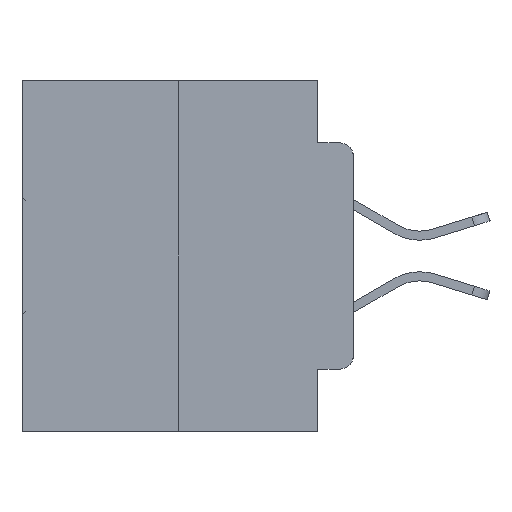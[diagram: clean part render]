
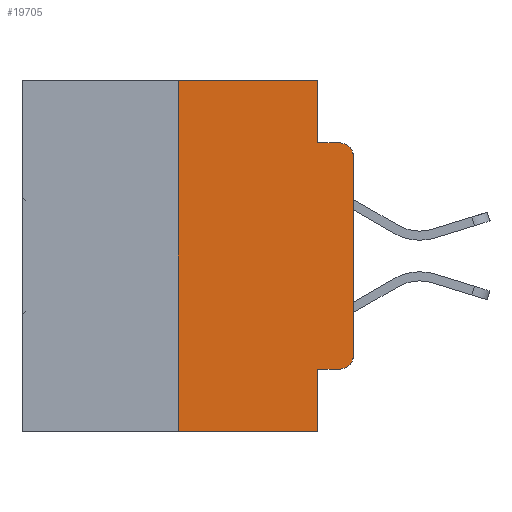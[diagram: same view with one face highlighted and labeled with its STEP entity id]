
A CAD part, left-side view. The second image highlights one B-rep face of the part: STEP entity #19705.
In plain terms, the highlighted planar face has unit normal (-1, 0, 0).
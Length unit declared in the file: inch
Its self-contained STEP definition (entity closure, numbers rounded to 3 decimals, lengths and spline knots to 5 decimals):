
#612 = VERTEX_POINT ( 'NONE', #26091 ) ;
#652 = EDGE_CURVE ( 'NONE', #20624, #612, #1993, .T. ) ;
#1341 = DIRECTION ( 'NONE',  ( 0., -1., 0. ) ) ;
#1953 = EDGE_CURVE ( 'NONE', #21382, #4278, #17547, .T. ) ;
#1993 = LINE ( 'NONE', #6471, #13071 ) ;
#2109 = CIRCLE ( 'NONE', #30244, 0.02 ) ;
#2311 = DIRECTION ( 'NONE',  ( 0., 0., -1. ) ) ;
#2316 = DIRECTION ( 'NONE',  ( 0., 0., -1. ) ) ;
#2980 = CARTESIAN_POINT ( 'NONE',  ( 0., 0.02, -0.1085 ) ) ;
#3185 = DIRECTION ( 'NONE',  ( 0., 0., 1. ) ) ;
#3675 = EDGE_CURVE ( 'NONE', #23677, #4278, #2109, .T. ) ;
#4153 = CIRCLE ( 'NONE', #27238, 0.02 ) ;
#4278 = VERTEX_POINT ( 'NONE', #30336 ) ;
#4322 = LINE ( 'NONE', #11674, #23348 ) ;
#4715 = VERTEX_POINT ( 'NONE', #14720 ) ;
#5131 = ORIENTED_EDGE ( 'NONE', *, *, #17957, .F. ) ;
#5342 = DIRECTION ( 'NONE',  ( -1., 0., 0. ) ) ;
#5421 = EDGE_CURVE ( 'NONE', #15825, #23677, #31014, .T. ) ;
#5577 = DIRECTION ( 'NONE',  ( 0., 0., -1. ) ) ;
#5592 = ORIENTED_EDGE ( 'NONE', *, *, #652, .T. ) ;
#5945 = AXIS2_PLACEMENT_3D ( 'NONE', #31873, #17349, #2316 ) ;
#6471 = CARTESIAN_POINT ( 'NONE',  ( 0., 0.473, -0.5 ) ) ;
#6844 = ORIENTED_EDGE ( 'NONE', *, *, #29112, .F. ) ;
#7915 = ORIENTED_EDGE ( 'NONE', *, *, #24277, .T. ) ;
#8422 = ORIENTED_EDGE ( 'NONE', *, *, #25894, .F. ) ;
#9498 = DIRECTION ( 'NONE',  ( 0., -1., 0. ) ) ;
#9536 = ORIENTED_EDGE ( 'NONE', *, *, #22632, .T. ) ;
#9885 = CARTESIAN_POINT ( 'NONE',  ( 0., 0.473, 0. ) ) ;
#11056 = VECTOR ( 'NONE', #2311, 39.37008 ) ;
#11674 = CARTESIAN_POINT ( 'NONE',  ( 0., 0.051, 0. ) ) ;
#12160 = VERTEX_POINT ( 'NONE', #20663 ) ;
#12467 = VERTEX_POINT ( 'NONE', #21724 ) ;
#12592 = CARTESIAN_POINT ( 'NONE',  ( 0., 0.25, -0.5 ) ) ;
#13071 = VECTOR ( 'NONE', #14023, 39.37008 ) ;
#13383 = DIRECTION ( 'NONE',  ( 0., 0., 1. ) ) ;
#13557 = ORIENTED_EDGE ( 'NONE', *, *, #3675, .T. ) ;
#14023 = DIRECTION ( 'NONE',  ( 0., -1., 0. ) ) ;
#14187 = DIRECTION ( 'NONE',  ( 0., 0., -1. ) ) ;
#14583 = ORIENTED_EDGE ( 'NONE', *, *, #1953, .F. ) ;
#14720 = CARTESIAN_POINT ( 'NONE',  ( 0., 0.051, -0.4115 ) ) ;
#14884 = CARTESIAN_POINT ( 'NONE',  ( 0., 0.051, 0. ) ) ;
#15825 = VERTEX_POINT ( 'NONE', #22467 ) ;
#15862 = VECTOR ( 'NONE', #22148, 39.37008 ) ;
#16589 = CARTESIAN_POINT ( 'NONE',  ( 0., 0., -0.1085 ) ) ;
#17349 = DIRECTION ( 'NONE',  ( 1., 0., 0. ) ) ;
#17547 = LINE ( 'NONE', #24125, #28156 ) ;
#17957 = EDGE_CURVE ( 'NONE', #12467, #12160, #22346, .T. ) ;
#18044 = CARTESIAN_POINT ( 'NONE',  ( 0., 0.051, -0.0885 ) ) ;
#19705 = ADVANCED_FACE ( 'NONE', ( #29414 ), #29444, .F. ) ;
#20195 = CARTESIAN_POINT ( 'NONE',  ( 0., 0.02, -0.3915 ) ) ;
#20419 = DIRECTION ( 'NONE',  ( -1., 0., 0. ) ) ;
#20471 = CARTESIAN_POINT ( 'NONE',  ( 0., 0.02, -0.4115 ) ) ;
#20607 = CARTESIAN_POINT ( 'NONE',  ( 0., 0.25, 0. ) ) ;
#20624 = VERTEX_POINT ( 'NONE', #12592 ) ;
#20645 = CARTESIAN_POINT ( 'NONE',  ( 0., 0., 0. ) ) ;
#20663 = CARTESIAN_POINT ( 'NONE',  ( 0., 0.051, 0. ) ) ;
#21220 = CARTESIAN_POINT ( 'NONE',  ( 0., 0.051, -0.4115 ) ) ;
#21382 = VERTEX_POINT ( 'NONE', #18044 ) ;
#21724 = CARTESIAN_POINT ( 'NONE',  ( 0., 0.25, 0. ) ) ;
#21937 = VECTOR ( 'NONE', #1341, 39.37008 ) ;
#22148 = DIRECTION ( 'NONE',  ( 0., -1., 0. ) ) ;
#22346 = LINE ( 'NONE', #9885, #15862 ) ;
#22467 = CARTESIAN_POINT ( 'NONE',  ( 0., 0., -0.3915 ) ) ;
#22632 = EDGE_CURVE ( 'NONE', #28074, #15825, #4153, .T. ) ;
#22663 = DIRECTION ( 'NONE',  ( 0., 0., -1. ) ) ;
#23348 = VECTOR ( 'NONE', #14187, 39.37008 ) ;
#23677 = VERTEX_POINT ( 'NONE', #16589 ) ;
#24125 = CARTESIAN_POINT ( 'NONE',  ( 0., 0.051, -0.0885 ) ) ;
#24277 = EDGE_CURVE ( 'NONE', #4715, #28074, #26865, .T. ) ;
#24638 = VECTOR ( 'NONE', #13383, 39.37008 ) ;
#24835 = EDGE_LOOP ( 'NONE', ( #28732, #13557, #14583, #6844, #5131, #31367, #5592, #8422, #7915, #9536 ) ) ;
#25894 = EDGE_CURVE ( 'NONE', #4715, #612, #4322, .T. ) ;
#26091 = CARTESIAN_POINT ( 'NONE',  ( 0., 0.051, -0.5 ) ) ;
#26865 = LINE ( 'NONE', #21220, #21937 ) ;
#27238 = AXIS2_PLACEMENT_3D ( 'NONE', #20195, #5342, #22663 ) ;
#27487 = EDGE_CURVE ( 'NONE', #20624, #12467, #27946, .T. ) ;
#27946 = LINE ( 'NONE', #20607, #28706 ) ;
#28074 = VERTEX_POINT ( 'NONE', #20471 ) ;
#28156 = VECTOR ( 'NONE', #9498, 39.37008 ) ;
#28706 = VECTOR ( 'NONE', #3185, 39.37008 ) ;
#28732 = ORIENTED_EDGE ( 'NONE', *, *, #5421, .T. ) ;
#29112 = EDGE_CURVE ( 'NONE', #12160, #21382, #31300, .T. ) ;
#29414 = FACE_OUTER_BOUND ( 'NONE', #24835, .T. ) ;
#29444 = PLANE ( 'NONE',  #5945 ) ;
#30244 = AXIS2_PLACEMENT_3D ( 'NONE', #2980, #20419, #5577 ) ;
#30336 = CARTESIAN_POINT ( 'NONE',  ( 0., 0.02, -0.0885 ) ) ;
#31014 = LINE ( 'NONE', #20645, #24638 ) ;
#31300 = LINE ( 'NONE', #14884, #11056 ) ;
#31367 = ORIENTED_EDGE ( 'NONE', *, *, #27487, .F. ) ;
#31873 = CARTESIAN_POINT ( 'NONE',  ( 0., 0.473, 0. ) ) ;
